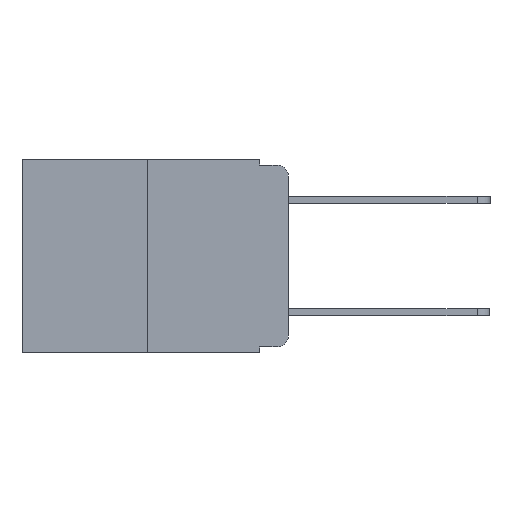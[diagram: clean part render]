
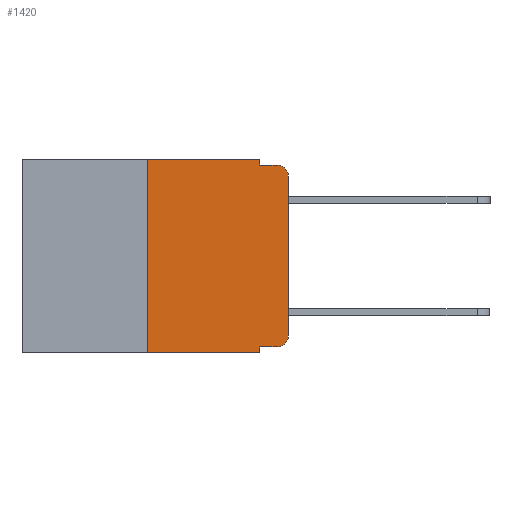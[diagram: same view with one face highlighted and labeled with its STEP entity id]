
A CAD part, left-side view. The second image highlights one B-rep face of the part: STEP entity #1420.
In plain terms, the highlighted planar face has unit normal (-1, 0, 0).
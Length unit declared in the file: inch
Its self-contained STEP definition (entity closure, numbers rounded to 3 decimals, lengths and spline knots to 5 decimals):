
#7 = CIRCLE ( 'NONE', #7638, 0.02 ) ;
#284 = EDGE_CURVE ( 'NONE', #2595, #10376, #7, .T. ) ;
#956 = VERTEX_POINT ( 'NONE', #14845 ) ;
#1004 = VECTOR ( 'NONE', #7074, 39.37008 ) ;
#1025 = ORIENTED_EDGE ( 'NONE', *, *, #9384, .F. ) ;
#1178 = EDGE_CURVE ( 'NONE', #956, #2595, #2756, .T. ) ;
#1420 = ADVANCED_FACE ( 'NONE', ( #12775 ), #14198, .F. ) ;
#1423 = LINE ( 'NONE', #9087, #7789 ) ;
#1590 = DIRECTION ( 'NONE',  ( 0., -1., 0. ) ) ;
#1601 = CARTESIAN_POINT ( 'NONE',  ( 0., 0., -0.03 ) ) ;
#1657 = ORIENTED_EDGE ( 'NONE', *, *, #14655, .F. ) ;
#1765 = DIRECTION ( 'NONE',  ( 0., -1., 0. ) ) ;
#1905 = VERTEX_POINT ( 'NONE', #12544 ) ;
#2012 = AXIS2_PLACEMENT_3D ( 'NONE', #3756, #15285, #2432 ) ;
#2029 = CARTESIAN_POINT ( 'NONE',  ( 0., 0.02, -0.313 ) ) ;
#2069 = CARTESIAN_POINT ( 'NONE',  ( 0., 0.02, -0.03 ) ) ;
#2339 = ORIENTED_EDGE ( 'NONE', *, *, #13872, .F. ) ;
#2432 = DIRECTION ( 'NONE',  ( 0., 0., -1. ) ) ;
#2595 = VERTEX_POINT ( 'NONE', #1601 ) ;
#2597 = VERTEX_POINT ( 'NONE', #10276 ) ;
#2747 = ORIENTED_EDGE ( 'NONE', *, *, #1178, .T. ) ;
#2756 = LINE ( 'NONE', #13091, #1004 ) ;
#2962 = VERTEX_POINT ( 'NONE', #12529 ) ;
#3407 = DIRECTION ( 'NONE',  ( 0., 0., -1. ) ) ;
#3419 = VECTOR ( 'NONE', #10899, 39.37008 ) ;
#3642 = LINE ( 'NONE', #3702, #15893 ) ;
#3702 = CARTESIAN_POINT ( 'NONE',  ( 0., 0.25, 0. ) ) ;
#3756 = CARTESIAN_POINT ( 'NONE',  ( 0., 0.473, 0. ) ) ;
#4446 = ORIENTED_EDGE ( 'NONE', *, *, #7302, .T. ) ;
#4771 = DIRECTION ( 'NONE',  ( 0., -1., 0. ) ) ;
#5043 = ORIENTED_EDGE ( 'NONE', *, *, #9182, .T. ) ;
#5830 = VERTEX_POINT ( 'NONE', #14297 ) ;
#5974 = ORIENTED_EDGE ( 'NONE', *, *, #10888, .F. ) ;
#6118 = CARTESIAN_POINT ( 'NONE',  ( 0., 0.25, -0.343 ) ) ;
#6197 = DIRECTION ( 'NONE',  ( 0., 0., 1. ) ) ;
#7074 = DIRECTION ( 'NONE',  ( 0., 0., 1. ) ) ;
#7217 = AXIS2_PLACEMENT_3D ( 'NONE', #2029, #10613, #3407 ) ;
#7302 = EDGE_CURVE ( 'NONE', #15830, #12386, #13777, .T. ) ;
#7638 = AXIS2_PLACEMENT_3D ( 'NONE', #2069, #8175, #12903 ) ;
#7789 = VECTOR ( 'NONE', #13864, 39.37008 ) ;
#7867 = CARTESIAN_POINT ( 'NONE',  ( 0., 0.051, -0.01 ) ) ;
#8175 = DIRECTION ( 'NONE',  ( -1., 0., 0. ) ) ;
#8923 = LINE ( 'NONE', #9227, #14835 ) ;
#9087 = CARTESIAN_POINT ( 'NONE',  ( 0., 0.051, 0. ) ) ;
#9182 = EDGE_CURVE ( 'NONE', #1905, #956, #15752, .T. ) ;
#9227 = CARTESIAN_POINT ( 'NONE',  ( 0., 0.473, 0. ) ) ;
#9384 = EDGE_CURVE ( 'NONE', #15830, #5830, #3642, .T. ) ;
#9651 = EDGE_LOOP ( 'NONE', ( #2747, #13539, #1657, #2339, #5974, #1025, #4446, #11512, #9855, #5043 ) ) ;
#9665 = EDGE_CURVE ( 'NONE', #2597, #1905, #9844, .T. ) ;
#9717 = CARTESIAN_POINT ( 'NONE',  ( 0., 0.051, -0.333 ) ) ;
#9741 = CARTESIAN_POINT ( 'NONE',  ( 0., 0.051, -0.343 ) ) ;
#9844 = LINE ( 'NONE', #9717, #3419 ) ;
#9855 = ORIENTED_EDGE ( 'NONE', *, *, #9665, .T. ) ;
#9973 = VECTOR ( 'NONE', #1590, 39.37008 ) ;
#10276 = CARTESIAN_POINT ( 'NONE',  ( 0., 0.051, -0.333 ) ) ;
#10337 = LINE ( 'NONE', #7867, #9973 ) ;
#10376 = VERTEX_POINT ( 'NONE', #11900 ) ;
#10613 = DIRECTION ( 'NONE',  ( -1., 0., 0. ) ) ;
#10860 = CARTESIAN_POINT ( 'NONE',  ( 0., 0.051, 0. ) ) ;
#10888 = EDGE_CURVE ( 'NONE', #5830, #11169, #8923, .T. ) ;
#10899 = DIRECTION ( 'NONE',  ( 0., -1., 0. ) ) ;
#11169 = VERTEX_POINT ( 'NONE', #10860 ) ;
#11336 = VECTOR ( 'NONE', #4771, 39.37008 ) ;
#11512 = ORIENTED_EDGE ( 'NONE', *, *, #12014, .F. ) ;
#11743 = DIRECTION ( 'NONE',  ( 0., 0., -1. ) ) ;
#11900 = CARTESIAN_POINT ( 'NONE',  ( 0., 0.02, -0.01 ) ) ;
#12014 = EDGE_CURVE ( 'NONE', #2597, #12386, #1423, .T. ) ;
#12386 = VERTEX_POINT ( 'NONE', #9741 ) ;
#12529 = CARTESIAN_POINT ( 'NONE',  ( 0., 0.051, -0.01 ) ) ;
#12544 = CARTESIAN_POINT ( 'NONE',  ( 0., 0.02, -0.333 ) ) ;
#12775 = FACE_OUTER_BOUND ( 'NONE', #9651, .T. ) ;
#12903 = DIRECTION ( 'NONE',  ( 0., 0., -1. ) ) ;
#12958 = CARTESIAN_POINT ( 'NONE',  ( 0., 0.051, 0. ) ) ;
#13091 = CARTESIAN_POINT ( 'NONE',  ( 0., 0., 0. ) ) ;
#13539 = ORIENTED_EDGE ( 'NONE', *, *, #284, .T. ) ;
#13777 = LINE ( 'NONE', #15444, #11336 ) ;
#13864 = DIRECTION ( 'NONE',  ( 0., 0., -1. ) ) ;
#13872 = EDGE_CURVE ( 'NONE', #11169, #2962, #15674, .T. ) ;
#14198 = PLANE ( 'NONE',  #2012 ) ;
#14297 = CARTESIAN_POINT ( 'NONE',  ( 0., 0.25, 0. ) ) ;
#14611 = VECTOR ( 'NONE', #11743, 39.37008 ) ;
#14655 = EDGE_CURVE ( 'NONE', #2962, #10376, #10337, .T. ) ;
#14835 = VECTOR ( 'NONE', #1765, 39.37008 ) ;
#14845 = CARTESIAN_POINT ( 'NONE',  ( 0., 0., -0.313 ) ) ;
#15285 = DIRECTION ( 'NONE',  ( 1., 0., 0. ) ) ;
#15444 = CARTESIAN_POINT ( 'NONE',  ( 0., 0.473, -0.343 ) ) ;
#15674 = LINE ( 'NONE', #12958, #14611 ) ;
#15752 = CIRCLE ( 'NONE', #7217, 0.02 ) ;
#15830 = VERTEX_POINT ( 'NONE', #6118 ) ;
#15893 = VECTOR ( 'NONE', #6197, 39.37008 ) ;
